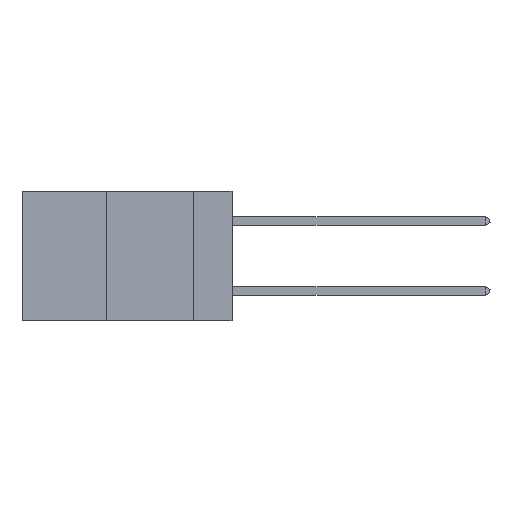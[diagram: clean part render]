
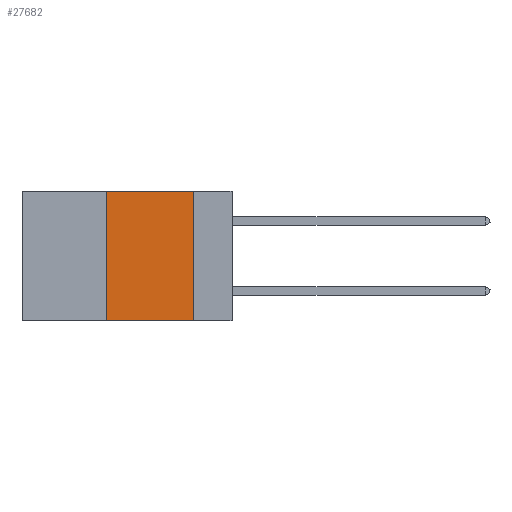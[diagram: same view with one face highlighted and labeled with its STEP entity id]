
A CAD part, left-side view. The second image highlights one B-rep face of the part: STEP entity #27682.
In plain terms, the highlighted planar face has unit normal (-1, 0, 0).
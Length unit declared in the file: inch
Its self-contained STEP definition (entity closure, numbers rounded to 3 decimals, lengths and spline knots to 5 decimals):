
#633 = LINE ( 'NONE', #9958, #5266 ) ;
#1977 = LINE ( 'NONE', #3476, #27460 ) ;
#2696 = EDGE_CURVE ( 'NONE', #23830, #30875, #25796, .T. ) ;
#3476 = CARTESIAN_POINT ( 'NONE',  ( 0., 0.6, 0. ) ) ;
#3786 = DIRECTION ( 'NONE',  ( 0., 0., -1. ) ) ;
#5266 = VECTOR ( 'NONE', #3786, 39.37008 ) ;
#5698 = CARTESIAN_POINT ( 'NONE',  ( 0., 0.11, -0.37 ) ) ;
#7793 = VERTEX_POINT ( 'NONE', #5698 ) ;
#8181 = DIRECTION ( 'NONE',  ( 0., 0., 1. ) ) ;
#8471 = CARTESIAN_POINT ( 'NONE',  ( 0., 0.36, 0. ) ) ;
#9161 = FACE_OUTER_BOUND ( 'NONE', #14986, .T. ) ;
#9958 = CARTESIAN_POINT ( 'NONE',  ( 0., 0.11, 0. ) ) ;
#10336 = EDGE_CURVE ( 'NONE', #30875, #18202, #1977, .T. ) ;
#10867 = CARTESIAN_POINT ( 'NONE',  ( 0., 0.6, -0.37 ) ) ;
#12951 = CARTESIAN_POINT ( 'NONE',  ( 0., 0.36, -0.37 ) ) ;
#13765 = CARTESIAN_POINT ( 'NONE',  ( 0., 0.6, 0. ) ) ;
#13894 = DIRECTION ( 'NONE',  ( 1., 0., 0. ) ) ;
#14986 = EDGE_LOOP ( 'NONE', ( #20375, #29798, #33045, #34430 ) ) ;
#16033 = VECTOR ( 'NONE', #8181, 39.37008 ) ;
#16833 = DIRECTION ( 'NONE',  ( 0., -1., 0. ) ) ;
#17999 = EDGE_CURVE ( 'NONE', #23830, #7793, #30806, .T. ) ;
#18202 = VERTEX_POINT ( 'NONE', #38012 ) ;
#18796 = EDGE_CURVE ( 'NONE', #18202, #7793, #633, .T. ) ;
#18813 = VECTOR ( 'NONE', #16833, 39.37008 ) ;
#20375 = ORIENTED_EDGE ( 'NONE', *, *, #18796, .F. ) ;
#23830 = VERTEX_POINT ( 'NONE', #12951 ) ;
#25437 = DIRECTION ( 'NONE',  ( 0., 0., -1. ) ) ;
#25678 = CARTESIAN_POINT ( 'NONE',  ( 0., 0.36, 0. ) ) ;
#25796 = LINE ( 'NONE', #25678, #16033 ) ;
#27460 = VECTOR ( 'NONE', #35441, 39.37008 ) ;
#27682 = ADVANCED_FACE ( 'NONE', ( #9161 ), #37302, .F. ) ;
#29798 = ORIENTED_EDGE ( 'NONE', *, *, #10336, .F. ) ;
#30806 = LINE ( 'NONE', #10867, #18813 ) ;
#30875 = VERTEX_POINT ( 'NONE', #8471 ) ;
#31389 = AXIS2_PLACEMENT_3D ( 'NONE', #13765, #13894, #25437 ) ;
#33045 = ORIENTED_EDGE ( 'NONE', *, *, #2696, .F. ) ;
#34430 = ORIENTED_EDGE ( 'NONE', *, *, #17999, .T. ) ;
#35441 = DIRECTION ( 'NONE',  ( 0., -1., 0. ) ) ;
#37302 = PLANE ( 'NONE',  #31389 ) ;
#38012 = CARTESIAN_POINT ( 'NONE',  ( 0., 0.11, 0. ) ) ;
